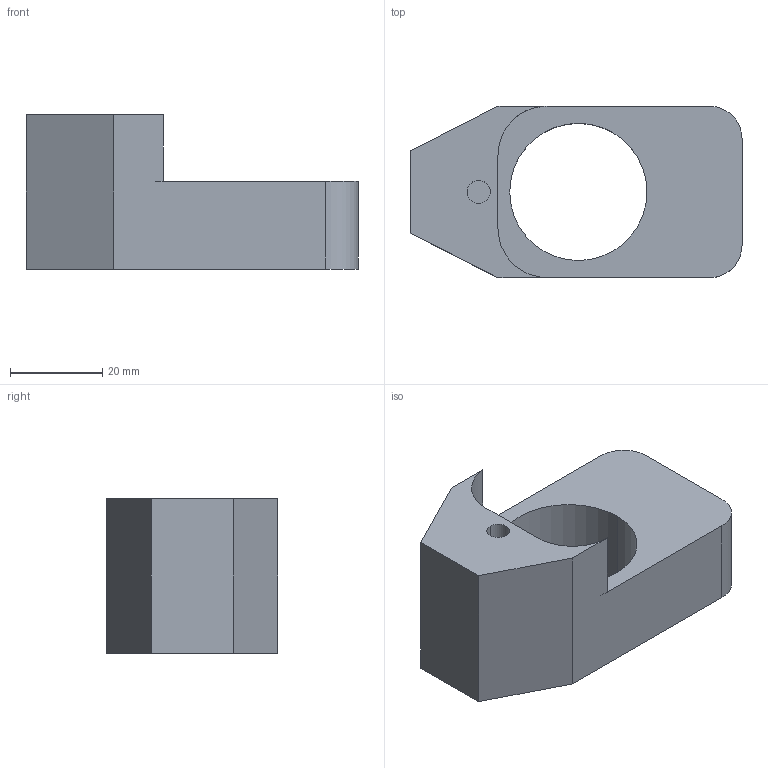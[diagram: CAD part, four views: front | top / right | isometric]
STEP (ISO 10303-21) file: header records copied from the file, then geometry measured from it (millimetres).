
FILE_DESCRIPTION (( 'STEP AP214' ), '1' );
FILE_NAME ('MAINSPRING_RETAINER.STEP', '2013-05-15T15:01:52', ( 'Asher' ), ( '' ), 'SwSTEP 2.0', 'SolidWorks 2013', '' );
FILE_SCHEMA (( 'AUTOMOTIVE_DESIGN' ));
Length unit declared in the file: inch
Products named in the file (1): MAINSPRING_RETAINER
Bounding box: 71.88 x 37.13 x 33.4 mm (x, y, z)
Volume: 41535.8 mm3; surface area: 11206.2 mm2
Topology: 1 solids, 1 shells, 21 faces, 53 edges, 35 vertices
Faces by surface type: plane 12, cylinder 9
Entity records: 681 total; most frequent: DIRECTION 115, CARTESIAN_POINT 110, ORIENTED_EDGE 106, EDGE_CURVE 53, AXIS2_PLACEMENT_3D 40, VECTOR 35, LINE 35, VERTEX_POINT 35
